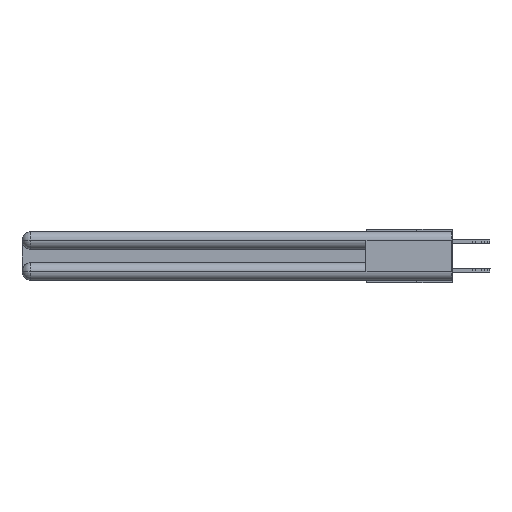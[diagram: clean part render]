
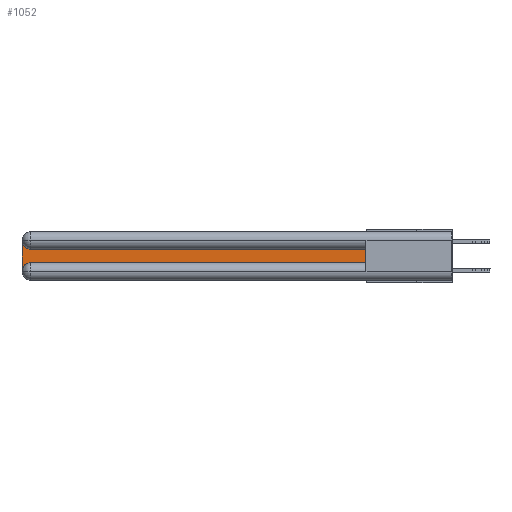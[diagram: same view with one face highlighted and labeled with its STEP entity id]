
A CAD part, left-side view. The second image highlights one B-rep face of the part: STEP entity #1052.
In plain terms, the highlighted planar face has unit normal (-1, 0, 0).
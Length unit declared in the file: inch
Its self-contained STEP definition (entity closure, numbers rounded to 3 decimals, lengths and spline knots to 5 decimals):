
#57 = LINE ( 'NONE', #11333, #14620 ) ;
#117 = LINE ( 'NONE', #22985, #20116 ) ;
#867 = VERTEX_POINT ( 'NONE', #24611 ) ;
#1052 = ADVANCED_FACE ( 'NONE', ( #21731 ), #16619, .F. ) ;
#1474 = CARTESIAN_POINT ( 'NONE',  ( 0.075, 3., -0.1225 ) ) ;
#1537 = CARTESIAN_POINT ( 'NONE',  ( 0.075, 0.6, -0.1225 ) ) ;
#1606 = CARTESIAN_POINT ( 'NONE',  ( 0.075, 0.6, -0.2175 ) ) ;
#1652 = LINE ( 'NONE', #1606, #18578 ) ;
#1840 = ORIENTED_EDGE ( 'NONE', *, *, #10674, .T. ) ;
#1941 = DIRECTION ( 'NONE',  ( 1., 0., 0. ) ) ;
#2025 = CARTESIAN_POINT ( 'NONE',  ( 0.075, 2.94, -0.2175 ) ) ;
#2657 = DIRECTION ( 'NONE',  ( 0., 0., -1. ) ) ;
#3098 = EDGE_CURVE ( 'NONE', #19479, #8666, #14175, .T. ) ;
#5175 = ORIENTED_EDGE ( 'NONE', *, *, #23674, .T. ) ;
#5487 = DIRECTION ( 'NONE',  ( 0., 0., 1. ) ) ;
#5979 = CARTESIAN_POINT ( 'NONE',  ( 0.075, 2.94, -0.2775 ) ) ;
#8008 = CARTESIAN_POINT ( 'NONE',  ( 0.075, 2.94, -0.0625 ) ) ;
#8210 = DIRECTION ( 'NONE',  ( 1., 0., 0. ) ) ;
#8666 = VERTEX_POINT ( 'NONE', #2025 ) ;
#10147 = DIRECTION ( 'NONE',  ( 0., 0., -1. ) ) ;
#10551 = ORIENTED_EDGE ( 'NONE', *, *, #26875, .T. ) ;
#10674 = EDGE_CURVE ( 'NONE', #17898, #19508, #117, .T. ) ;
#10981 = DIRECTION ( 'NONE',  ( 0., 0., -1. ) ) ;
#11333 = CARTESIAN_POINT ( 'NONE',  ( 0.075, 3., -0.2175 ) ) ;
#12637 = DIRECTION ( 'NONE',  ( 0., 0., -1. ) ) ;
#14175 = CIRCLE ( 'NONE', #27510, 0.06 ) ;
#14620 = VECTOR ( 'NONE', #2657, 39.37008 ) ;
#14661 = DIRECTION ( 'NONE',  ( 0., -1., 0. ) ) ;
#15886 = CARTESIAN_POINT ( 'NONE',  ( 0.075, 0.6, -0.2175 ) ) ;
#16381 = CARTESIAN_POINT ( 'NONE',  ( 0.075, 2.94, -0.1225 ) ) ;
#16619 = PLANE ( 'NONE',  #22236 ) ;
#16676 = DIRECTION ( 'NONE',  ( 0., 1., 0. ) ) ;
#17434 = VERTEX_POINT ( 'NONE', #16381 ) ;
#17712 = CIRCLE ( 'NONE', #21251, 0.06 ) ;
#17898 = VERTEX_POINT ( 'NONE', #15886 ) ;
#18401 = ORIENTED_EDGE ( 'NONE', *, *, #21449, .T. ) ;
#18514 = VECTOR ( 'NONE', #16676, 39.37008 ) ;
#18578 = VECTOR ( 'NONE', #14661, 39.37008 ) ;
#18699 = EDGE_CURVE ( 'NONE', #19508, #17434, #20898, .T. ) ;
#19479 = VERTEX_POINT ( 'NONE', #21500 ) ;
#19508 = VERTEX_POINT ( 'NONE', #28021 ) ;
#20116 = VECTOR ( 'NONE', #5487, 39.37008 ) ;
#20898 = LINE ( 'NONE', #1537, #18514 ) ;
#21251 = AXIS2_PLACEMENT_3D ( 'NONE', #8008, #1941, #10981 ) ;
#21449 = EDGE_CURVE ( 'NONE', #867, #19479, #57, .T. ) ;
#21489 = ORIENTED_EDGE ( 'NONE', *, *, #18699, .T. ) ;
#21500 = CARTESIAN_POINT ( 'NONE',  ( 0.075, 3., -0.2775 ) ) ;
#21731 = FACE_OUTER_BOUND ( 'NONE', #22396, .T. ) ;
#22236 = AXIS2_PLACEMENT_3D ( 'NONE', #1474, #25238, #10147 ) ;
#22396 = EDGE_LOOP ( 'NONE', ( #21489, #10551, #18401, #22613, #5175, #1840 ) ) ;
#22613 = ORIENTED_EDGE ( 'NONE', *, *, #3098, .T. ) ;
#22985 = CARTESIAN_POINT ( 'NONE',  ( 0.075, 0.6, -0.2175 ) ) ;
#23674 = EDGE_CURVE ( 'NONE', #8666, #17898, #1652, .T. ) ;
#24611 = CARTESIAN_POINT ( 'NONE',  ( 0.075, 3., -0.0625 ) ) ;
#25238 = DIRECTION ( 'NONE',  ( 1., 0., 0. ) ) ;
#26875 = EDGE_CURVE ( 'NONE', #17434, #867, #17712, .T. ) ;
#27510 = AXIS2_PLACEMENT_3D ( 'NONE', #5979, #8210, #12637 ) ;
#28021 = CARTESIAN_POINT ( 'NONE',  ( 0.075, 0.6, -0.1225 ) ) ;
